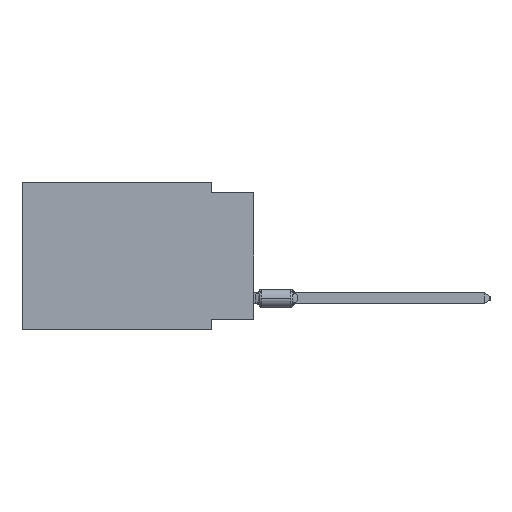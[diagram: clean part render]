
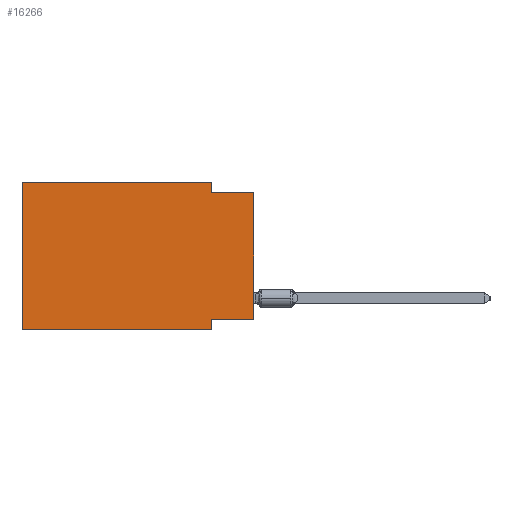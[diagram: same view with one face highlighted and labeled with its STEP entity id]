
A CAD part, left-side view. The second image highlights one B-rep face of the part: STEP entity #16266.
In plain terms, the highlighted planar face has unit normal (-1, 0, 0).
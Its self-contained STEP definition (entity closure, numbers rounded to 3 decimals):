
#1079 = LINE ( 'NONE', #38074, #29047 ) ;
#1739 = PLANE ( 'NONE',  #6654 ) ;
#3163 = CARTESIAN_POINT ( 'NONE',  ( 0., 2.54, -8.89 ) ) ;
#3727 = ORIENTED_EDGE ( 'NONE', *, *, #65204, .T. ) ;
#5278 = EDGE_CURVE ( 'NONE', #30330, #31113, #38699, .T. ) ;
#5545 = CARTESIAN_POINT ( 'NONE',  ( 0., 0., -8.255 ) ) ;
#6585 = VERTEX_POINT ( 'NONE', #5545 ) ;
#6654 = AXIS2_PLACEMENT_3D ( 'NONE', #55194, #28776, #33583 ) ;
#7552 = FACE_OUTER_BOUND ( 'NONE', #57011, .T. ) ;
#7922 = VERTEX_POINT ( 'NONE', #41063 ) ;
#8731 = ORIENTED_EDGE ( 'NONE', *, *, #38342, .T. ) ;
#9168 = CARTESIAN_POINT ( 'NONE',  ( 0., 0., 0. ) ) ;
#10779 = EDGE_CURVE ( 'NONE', #66931, #7922, #67171, .T. ) ;
#11565 = EDGE_CURVE ( 'NONE', #7922, #30330, #62743, .T. ) ;
#12205 = LINE ( 'NONE', #43056, #36741 ) ;
#14120 = LINE ( 'NONE', #3163, #63958 ) ;
#14951 = VECTOR ( 'NONE', #25953, 1000. ) ;
#15766 = DIRECTION ( 'NONE',  ( 0., 0., -1. ) ) ;
#16266 = ADVANCED_FACE ( 'NONE', ( #7552 ), #1739, .F. ) ;
#21479 = VERTEX_POINT ( 'NONE', #67121 ) ;
#21635 = LINE ( 'NONE', #22308, #41608 ) ;
#21972 = DIRECTION ( 'NONE',  ( 0., 0., 1. ) ) ;
#22308 = CARTESIAN_POINT ( 'NONE',  ( 0., 13.97, -8.89 ) ) ;
#22895 = CARTESIAN_POINT ( 'NONE',  ( 0., 13.97, 0. ) ) ;
#23892 = CARTESIAN_POINT ( 'NONE',  ( 0., 2.54, -8.255 ) ) ;
#25716 = VECTOR ( 'NONE', #59619, 1000. ) ;
#25953 = DIRECTION ( 'NONE',  ( 0., -1., 0. ) ) ;
#27263 = DIRECTION ( 'NONE',  ( 0., 1., 0. ) ) ;
#28776 = DIRECTION ( 'NONE',  ( 1., 0., 0. ) ) ;
#29047 = VECTOR ( 'NONE', #21972, 1000. ) ;
#29734 = EDGE_CURVE ( 'NONE', #6585, #62714, #12205, .T. ) ;
#30039 = EDGE_CURVE ( 'NONE', #51702, #66931, #1079, .T. ) ;
#30330 = VERTEX_POINT ( 'NONE', #55878 ) ;
#30679 = CARTESIAN_POINT ( 'NONE',  ( 0., 13.97, -8.89 ) ) ;
#31113 = VERTEX_POINT ( 'NONE', #36967 ) ;
#33583 = DIRECTION ( 'NONE',  ( 0., 0., -1. ) ) ;
#34241 = CARTESIAN_POINT ( 'NONE',  ( 0., 0., -0.635 ) ) ;
#34336 = DIRECTION ( 'NONE',  ( 0., 0., -1. ) ) ;
#36741 = VECTOR ( 'NONE', #27263, 1000. ) ;
#36967 = CARTESIAN_POINT ( 'NONE',  ( 0., 0., -0.635 ) ) ;
#37945 = VECTOR ( 'NONE', #56465, 1000. ) ;
#38074 = CARTESIAN_POINT ( 'NONE',  ( 0., 13.97, 0. ) ) ;
#38342 = EDGE_CURVE ( 'NONE', #6585, #31113, #56121, .T. ) ;
#38699 = LINE ( 'NONE', #34241, #25716 ) ;
#41063 = CARTESIAN_POINT ( 'NONE',  ( 0., 2.54, 0. ) ) ;
#41608 = VECTOR ( 'NONE', #63480, 1000. ) ;
#43056 = CARTESIAN_POINT ( 'NONE',  ( 0., 0., -8.255 ) ) ;
#43156 = CARTESIAN_POINT ( 'NONE',  ( 0., 2.54, 0. ) ) ;
#44256 = ORIENTED_EDGE ( 'NONE', *, *, #10779, .F. ) ;
#45642 = ORIENTED_EDGE ( 'NONE', *, *, #30039, .F. ) ;
#46576 = CARTESIAN_POINT ( 'NONE',  ( 0., 13.97, 0. ) ) ;
#47155 = ORIENTED_EDGE ( 'NONE', *, *, #29734, .F. ) ;
#51702 = VERTEX_POINT ( 'NONE', #30679 ) ;
#55194 = CARTESIAN_POINT ( 'NONE',  ( 0., 13.97, 0. ) ) ;
#55327 = ORIENTED_EDGE ( 'NONE', *, *, #11565, .F. ) ;
#55878 = CARTESIAN_POINT ( 'NONE',  ( 0., 2.54, -0.635 ) ) ;
#56121 = LINE ( 'NONE', #9168, #37945 ) ;
#56465 = DIRECTION ( 'NONE',  ( 0., 0., 1. ) ) ;
#57011 = EDGE_LOOP ( 'NONE', ( #8731, #57373, #55327, #44256, #45642, #3727, #57168, #47155 ) ) ;
#57168 = ORIENTED_EDGE ( 'NONE', *, *, #60486, .F. ) ;
#57373 = ORIENTED_EDGE ( 'NONE', *, *, #5278, .F. ) ;
#59619 = DIRECTION ( 'NONE',  ( 0., -1., 0. ) ) ;
#60486 = EDGE_CURVE ( 'NONE', #62714, #21479, #14120, .T. ) ;
#62714 = VERTEX_POINT ( 'NONE', #23892 ) ;
#62743 = LINE ( 'NONE', #43156, #66497 ) ;
#63480 = DIRECTION ( 'NONE',  ( 0., -1., 0. ) ) ;
#63958 = VECTOR ( 'NONE', #34336, 1000. ) ;
#65204 = EDGE_CURVE ( 'NONE', #51702, #21479, #21635, .T. ) ;
#66497 = VECTOR ( 'NONE', #15766, 1000. ) ;
#66931 = VERTEX_POINT ( 'NONE', #22895 ) ;
#67121 = CARTESIAN_POINT ( 'NONE',  ( 0., 2.54, -8.89 ) ) ;
#67171 = LINE ( 'NONE', #46576, #14951 ) ;
